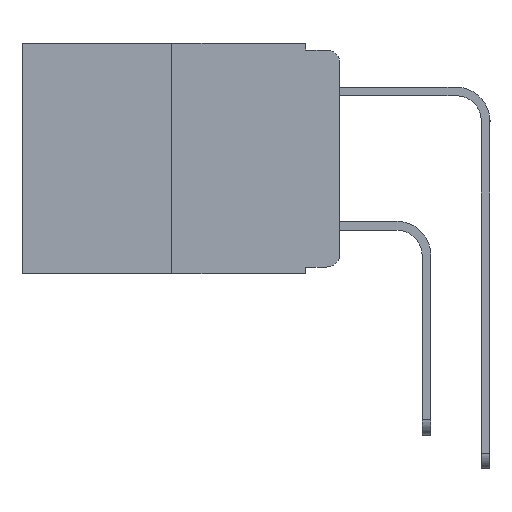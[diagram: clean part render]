
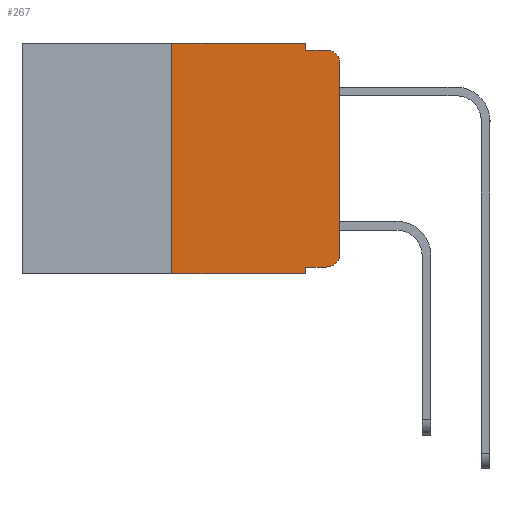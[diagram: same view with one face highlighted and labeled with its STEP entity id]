
A CAD part, left-side view. The second image highlights one B-rep face of the part: STEP entity #267.
In plain terms, the highlighted planar face has unit normal (-1, 0, 0).
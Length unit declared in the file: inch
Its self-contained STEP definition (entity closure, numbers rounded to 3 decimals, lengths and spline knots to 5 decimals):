
#20 = FACE_OUTER_BOUND ( 'NONE', #11341, .T. ) ;
#267 = ADVANCED_FACE ( 'NONE', ( #20 ), #9404, .F. ) ;
#664 = VERTEX_POINT ( 'NONE', #11174 ) ;
#722 = CARTESIAN_POINT ( 'NONE',  ( 0., 0.02, -0.313 ) ) ;
#1049 = EDGE_CURVE ( 'NONE', #9055, #13565, #8929, .T. ) ;
#1327 = CIRCLE ( 'NONE', #5145, 0.02 ) ;
#1333 = CIRCLE ( 'NONE', #13252, 0.02 ) ;
#1498 = LINE ( 'NONE', #14595, #9248 ) ;
#1549 = ORIENTED_EDGE ( 'NONE', *, *, #18853, .F. ) ;
#2169 = CARTESIAN_POINT ( 'NONE',  ( 0., 0., -0.313 ) ) ;
#2192 = EDGE_CURVE ( 'NONE', #12556, #13565, #1333, .T. ) ;
#2440 = DIRECTION ( 'NONE',  ( 0., 0., -1. ) ) ;
#2577 = VECTOR ( 'NONE', #3200, 39.37008 ) ;
#3200 = DIRECTION ( 'NONE',  ( 0., 0., -1. ) ) ;
#3300 = EDGE_CURVE ( 'NONE', #4685, #12556, #11137, .T. ) ;
#3321 = VERTEX_POINT ( 'NONE', #13738 ) ;
#3339 = CARTESIAN_POINT ( 'NONE',  ( 0., 0.051, 0. ) ) ;
#3889 = CARTESIAN_POINT ( 'NONE',  ( 0., 0.02, -0.03 ) ) ;
#4685 = VERTEX_POINT ( 'NONE', #2169 ) ;
#4782 = ORIENTED_EDGE ( 'NONE', *, *, #19658, .F. ) ;
#4940 = VECTOR ( 'NONE', #17817, 39.37008 ) ;
#5145 = AXIS2_PLACEMENT_3D ( 'NONE', #722, #11568, #2440 ) ;
#5242 = EDGE_CURVE ( 'NONE', #9683, #9440, #17058, .T. ) ;
#5368 = VECTOR ( 'NONE', #9738, 39.37008 ) ;
#5373 = CARTESIAN_POINT ( 'NONE',  ( 0., 0.051, -0.01 ) ) ;
#5429 = DIRECTION ( 'NONE',  ( 0., 0., -1. ) ) ;
#5755 = LINE ( 'NONE', #15471, #16787 ) ;
#7340 = CARTESIAN_POINT ( 'NONE',  ( 0., 0.051, 0. ) ) ;
#7583 = VECTOR ( 'NONE', #18738, 39.37008 ) ;
#8013 = DIRECTION ( 'NONE',  ( 0., -1., 0. ) ) ;
#8339 = ORIENTED_EDGE ( 'NONE', *, *, #2192, .T. ) ;
#8929 = LINE ( 'NONE', #5373, #5368 ) ;
#8974 = LINE ( 'NONE', #7340, #4940 ) ;
#9055 = VERTEX_POINT ( 'NONE', #11742 ) ;
#9102 = AXIS2_PLACEMENT_3D ( 'NONE', #14479, #14369, #14412 ) ;
#9248 = VECTOR ( 'NONE', #18986, 39.37008 ) ;
#9404 = PLANE ( 'NONE',  #9102 ) ;
#9440 = VERTEX_POINT ( 'NONE', #11023 ) ;
#9683 = VERTEX_POINT ( 'NONE', #17482 ) ;
#9738 = DIRECTION ( 'NONE',  ( 0., -1., 0. ) ) ;
#10040 = VERTEX_POINT ( 'NONE', #13814 ) ;
#10690 = ORIENTED_EDGE ( 'NONE', *, *, #5242, .T. ) ;
#11023 = CARTESIAN_POINT ( 'NONE',  ( 0., 0.051, -0.343 ) ) ;
#11137 = LINE ( 'NONE', #18110, #18550 ) ;
#11174 = CARTESIAN_POINT ( 'NONE',  ( 0., 0.02, -0.333 ) ) ;
#11341 = EDGE_LOOP ( 'NONE', ( #11841, #8339, #16297, #4782, #1549, #18105, #10690, #18558, #18345, #14912 ) ) ;
#11390 = VERTEX_POINT ( 'NONE', #18969 ) ;
#11568 = DIRECTION ( 'NONE',  ( -1., 0., 0. ) ) ;
#11569 = LINE ( 'NONE', #14337, #7583 ) ;
#11742 = CARTESIAN_POINT ( 'NONE',  ( 0., 0.051, -0.01 ) ) ;
#11841 = ORIENTED_EDGE ( 'NONE', *, *, #3300, .T. ) ;
#12556 = VERTEX_POINT ( 'NONE', #14149 ) ;
#13252 = AXIS2_PLACEMENT_3D ( 'NONE', #3889, #14443, #5429 ) ;
#13565 = VERTEX_POINT ( 'NONE', #19036 ) ;
#13671 = DIRECTION ( 'NONE',  ( 0., 0., 1. ) ) ;
#13734 = LINE ( 'NONE', #3339, #2577 ) ;
#13738 = CARTESIAN_POINT ( 'NONE',  ( 0., 0.051, 0. ) ) ;
#13814 = CARTESIAN_POINT ( 'NONE',  ( 0., 0.051, -0.333 ) ) ;
#14149 = CARTESIAN_POINT ( 'NONE',  ( 0., 0., -0.03 ) ) ;
#14337 = CARTESIAN_POINT ( 'NONE',  ( 0., 0.25, 0. ) ) ;
#14369 = DIRECTION ( 'NONE',  ( 1., 0., 0. ) ) ;
#14412 = DIRECTION ( 'NONE',  ( 0., 0., -1. ) ) ;
#14443 = DIRECTION ( 'NONE',  ( -1., 0., 0. ) ) ;
#14479 = CARTESIAN_POINT ( 'NONE',  ( 0., 0.473, 0. ) ) ;
#14595 = CARTESIAN_POINT ( 'NONE',  ( 0., 0.473, 0. ) ) ;
#14912 = ORIENTED_EDGE ( 'NONE', *, *, #15791, .T. ) ;
#15471 = CARTESIAN_POINT ( 'NONE',  ( 0., 0.051, -0.333 ) ) ;
#15625 = CARTESIAN_POINT ( 'NONE',  ( 0., 0.473, -0.343 ) ) ;
#15791 = EDGE_CURVE ( 'NONE', #664, #4685, #1327, .T. ) ;
#16297 = ORIENTED_EDGE ( 'NONE', *, *, #1049, .F. ) ;
#16605 = VECTOR ( 'NONE', #17154, 39.37008 ) ;
#16771 = EDGE_CURVE ( 'NONE', #10040, #664, #5755, .T. ) ;
#16787 = VECTOR ( 'NONE', #8013, 39.37008 ) ;
#17058 = LINE ( 'NONE', #15625, #16605 ) ;
#17154 = DIRECTION ( 'NONE',  ( 0., -1., 0. ) ) ;
#17482 = CARTESIAN_POINT ( 'NONE',  ( 0., 0.25, -0.343 ) ) ;
#17723 = EDGE_CURVE ( 'NONE', #10040, #9440, #13734, .T. ) ;
#17817 = DIRECTION ( 'NONE',  ( 0., 0., -1. ) ) ;
#18105 = ORIENTED_EDGE ( 'NONE', *, *, #18705, .F. ) ;
#18110 = CARTESIAN_POINT ( 'NONE',  ( 0., 0., 0. ) ) ;
#18345 = ORIENTED_EDGE ( 'NONE', *, *, #16771, .T. ) ;
#18550 = VECTOR ( 'NONE', #13671, 39.37008 ) ;
#18558 = ORIENTED_EDGE ( 'NONE', *, *, #17723, .F. ) ;
#18705 = EDGE_CURVE ( 'NONE', #9683, #11390, #11569, .T. ) ;
#18738 = DIRECTION ( 'NONE',  ( 0., 0., 1. ) ) ;
#18853 = EDGE_CURVE ( 'NONE', #11390, #3321, #1498, .T. ) ;
#18969 = CARTESIAN_POINT ( 'NONE',  ( 0., 0.25, 0. ) ) ;
#18986 = DIRECTION ( 'NONE',  ( 0., -1., 0. ) ) ;
#19036 = CARTESIAN_POINT ( 'NONE',  ( 0., 0.02, -0.01 ) ) ;
#19658 = EDGE_CURVE ( 'NONE', #3321, #9055, #8974, .T. ) ;
